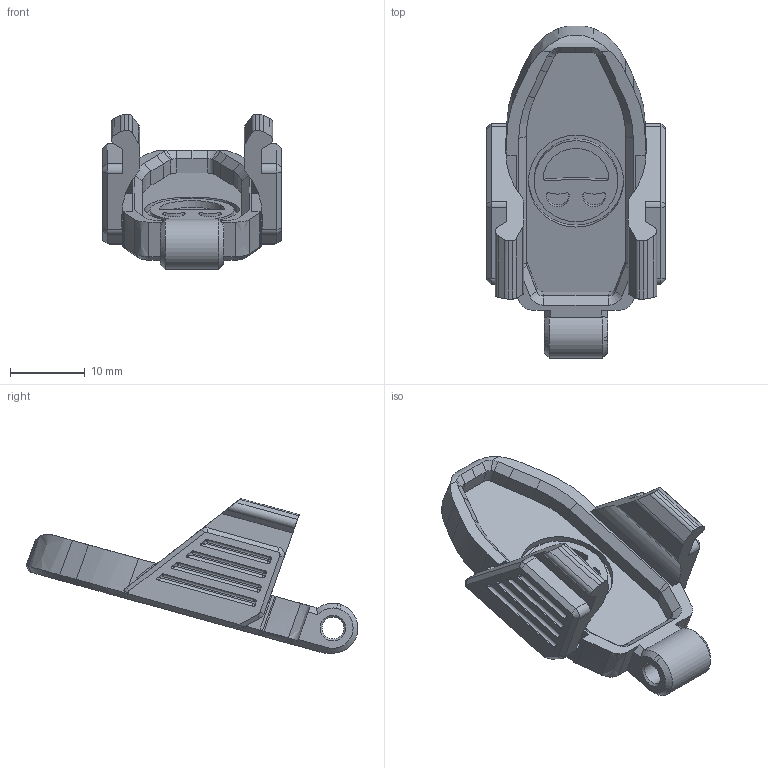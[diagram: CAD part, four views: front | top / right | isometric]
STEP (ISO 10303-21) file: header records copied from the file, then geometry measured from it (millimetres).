
FILE_DESCRIPTION(/* description */ (''),/* implementation_level */ '2;1');
FILE_NAME(/* name */ 'Grip Storage Hatch.step',/* time_stamp */ '2021-05-07T03:06:52-04:00',/* author */ (''),/* organization */ (''),/* preprocessor_version */ 'ST-DEVELOPER v18.1',/* originating_system */ 'Autodesk Translation Framework v10.6.0.1341',/* authorisation */ '');
FILE_SCHEMA (('AUTOMOTIVE_DESIGN { 1 0 10303 214 3 1 1 }'));
Length unit declared in the file: millimetre
Products named in the file (1): Grip Storage Hatch
Bounding box: 23.93 x 44.39 x 20.7 mm (x, y, z)
Volume: 3643.6 mm3; surface area: 3530 mm2
Topology: 1 solids, 1 shells, 354 faces, 897 edges, 526 vertices
Faces by surface type: plane 138, cylinder 112, bspline 84, cone 20
Full cylindrical faces by diameter (mm): 2.9 x1, 11.221 x1, 12.721 x1
Entity records: 11924 total; most frequent: CARTESIAN_POINT 3929, ORIENTED_EDGE 1730, DIRECTION 1518, EDGE_CURVE 865, VERTEX_POINT 526, AXIS2_PLACEMENT_3D 513, LINE 492, VECTOR 492
